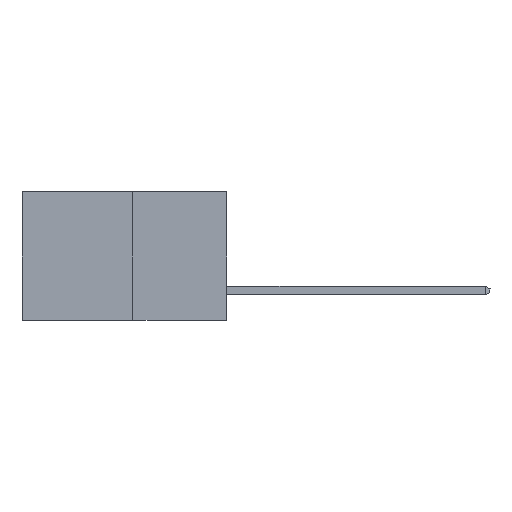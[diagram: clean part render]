
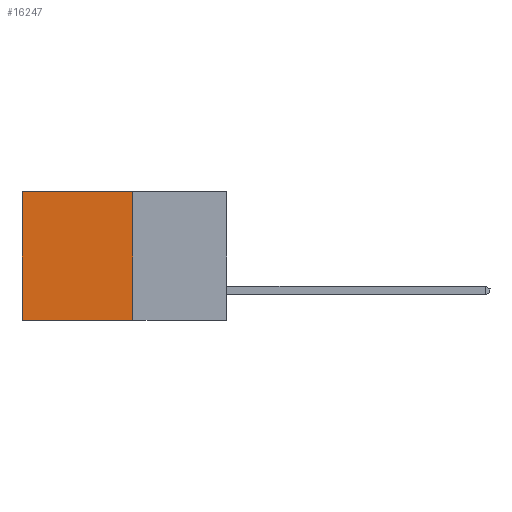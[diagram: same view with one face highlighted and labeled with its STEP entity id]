
A CAD part, left-side view. The second image highlights one B-rep face of the part: STEP entity #16247.
In plain terms, the highlighted planar face has unit normal (-1, 0, 0).
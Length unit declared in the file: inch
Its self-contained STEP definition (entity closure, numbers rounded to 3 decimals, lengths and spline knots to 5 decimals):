
#746 = CARTESIAN_POINT ( 'NONE',  ( 0.277, 0.27, 0. ) ) ;
#1024 = AXIS2_PLACEMENT_3D ( 'NONE', #10518, #2196, #11865 ) ;
#1502 = DIRECTION ( 'NONE',  ( 0., 0., -1. ) ) ;
#2070 = EDGE_CURVE ( 'NONE', #6381, #7392, #15717, .T. ) ;
#2196 = DIRECTION ( 'NONE',  ( 1., 0., 0. ) ) ;
#2656 = LINE ( 'NONE', #6134, #3116 ) ;
#3116 = VECTOR ( 'NONE', #6112, 39.37008 ) ;
#3987 = EDGE_CURVE ( 'NONE', #7392, #11987, #9828, .T. ) ;
#4182 = EDGE_CURVE ( 'NONE', #12196, #11987, #2656, .T. ) ;
#4789 = CARTESIAN_POINT ( 'NONE',  ( 0.277, 0.27, 0. ) ) ;
#5427 = VECTOR ( 'NONE', #1502, 39.37008 ) ;
#6112 = DIRECTION ( 'NONE',  ( 0., 0., -1. ) ) ;
#6134 = CARTESIAN_POINT ( 'NONE',  ( 0.277, 0.59, -0.37 ) ) ;
#6381 = VERTEX_POINT ( 'NONE', #746 ) ;
#7392 = VERTEX_POINT ( 'NONE', #14350 ) ;
#7987 = DIRECTION ( 'NONE',  ( 0., 1., 0. ) ) ;
#8065 = CARTESIAN_POINT ( 'NONE',  ( 0.277, 0.27, -0.37 ) ) ;
#8626 = CARTESIAN_POINT ( 'NONE',  ( 0.277, 0.59, -0.37 ) ) ;
#9023 = CARTESIAN_POINT ( 'NONE',  ( 0.277, 0.59, 0. ) ) ;
#9828 = LINE ( 'NONE', #8065, #16032 ) ;
#9898 = LINE ( 'NONE', #4789, #13899 ) ;
#10518 = CARTESIAN_POINT ( 'NONE',  ( 0.277, 0.27, -0.37 ) ) ;
#11524 = ORIENTED_EDGE ( 'NONE', *, *, #3987, .F. ) ;
#11865 = DIRECTION ( 'NONE',  ( 0., 0., -1. ) ) ;
#11987 = VERTEX_POINT ( 'NONE', #8626 ) ;
#12196 = VERTEX_POINT ( 'NONE', #9023 ) ;
#13017 = EDGE_CURVE ( 'NONE', #6381, #12196, #9898, .T. ) ;
#13229 = FACE_OUTER_BOUND ( 'NONE', #15867, .T. ) ;
#13899 = VECTOR ( 'NONE', #15575, 39.37008 ) ;
#14350 = CARTESIAN_POINT ( 'NONE',  ( 0.277, 0.27, -0.37 ) ) ;
#15441 = ORIENTED_EDGE ( 'NONE', *, *, #2070, .F. ) ;
#15575 = DIRECTION ( 'NONE',  ( 0., 1., 0. ) ) ;
#15717 = LINE ( 'NONE', #16545, #5427 ) ;
#15844 = ORIENTED_EDGE ( 'NONE', *, *, #13017, .T. ) ;
#15867 = EDGE_LOOP ( 'NONE', ( #17627, #11524, #15441, #15844 ) ) ;
#16032 = VECTOR ( 'NONE', #7987, 39.37008 ) ;
#16247 = ADVANCED_FACE ( 'NONE', ( #13229 ), #17049, .F. ) ;
#16545 = CARTESIAN_POINT ( 'NONE',  ( 0.277, 0.27, -0.37 ) ) ;
#17049 = PLANE ( 'NONE',  #1024 ) ;
#17627 = ORIENTED_EDGE ( 'NONE', *, *, #4182, .T. ) ;
